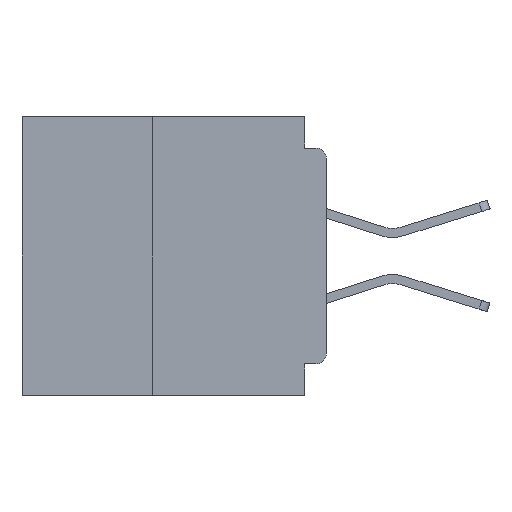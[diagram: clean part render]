
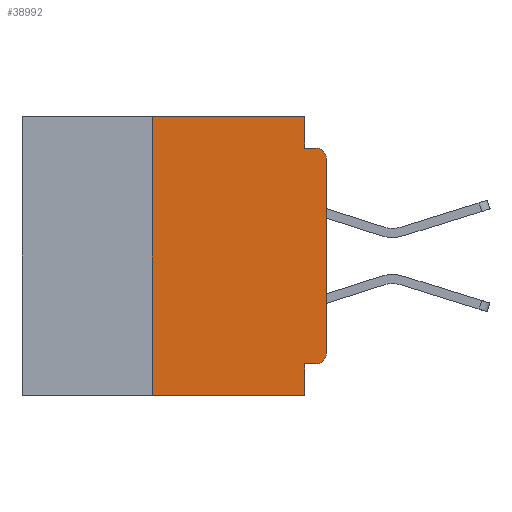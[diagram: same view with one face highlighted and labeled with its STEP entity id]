
A CAD part, left-side view. The second image highlights one B-rep face of the part: STEP entity #38992.
In plain terms, the highlighted planar face has unit normal (-1, 0, 0).
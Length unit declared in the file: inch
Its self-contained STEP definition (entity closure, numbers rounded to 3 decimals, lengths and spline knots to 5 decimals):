
#141 = CARTESIAN_POINT ( 'NONE',  ( 0., 0., -0.06 ) ) ;
#2053 = EDGE_CURVE ( 'NONE', #21252, #15218, #48424, .T. ) ;
#2383 = ORIENTED_EDGE ( 'NONE', *, *, #46104, .F. ) ;
#2386 = VERTEX_POINT ( 'NONE', #37650 ) ;
#2969 = DIRECTION ( 'NONE',  ( 0., 0., -1. ) ) ;
#3203 = AXIS2_PLACEMENT_3D ( 'NONE', #31301, #7996, #35089 ) ;
#5048 = VECTOR ( 'NONE', #17751, 39.37008 ) ;
#5997 = EDGE_CURVE ( 'NONE', #2386, #42788, #24803, .T. ) ;
#6348 = EDGE_CURVE ( 'NONE', #21252, #23633, #40868, .T. ) ;
#6538 = VECTOR ( 'NONE', #2969, 39.37008 ) ;
#7996 = DIRECTION ( 'NONE',  ( -1., 0., 0. ) ) ;
#8627 = CARTESIAN_POINT ( 'NONE',  ( 0., 0.031, -0.4 ) ) ;
#9634 = VERTEX_POINT ( 'NONE', #15767 ) ;
#10003 = CARTESIAN_POINT ( 'NONE',  ( 0., 0., 0. ) ) ;
#10216 = ORIENTED_EDGE ( 'NONE', *, *, #6348, .F. ) ;
#11369 = CARTESIAN_POINT ( 'NONE',  ( 0., 0.25, -0.4 ) ) ;
#11810 = PLANE ( 'NONE',  #15369 ) ;
#14421 = VECTOR ( 'NONE', #28930, 39.37008 ) ;
#14521 = ORIENTED_EDGE ( 'NONE', *, *, #5997, .F. ) ;
#14893 = CARTESIAN_POINT ( 'NONE',  ( 0., 0.25, 0. ) ) ;
#15218 = VERTEX_POINT ( 'NONE', #8627 ) ;
#15369 = AXIS2_PLACEMENT_3D ( 'NONE', #31027, #38784, #15764 ) ;
#15726 = LINE ( 'NONE', #18383, #6538 ) ;
#15750 = VERTEX_POINT ( 'NONE', #27182 ) ;
#15764 = DIRECTION ( 'NONE',  ( 0., 0., -1. ) ) ;
#15767 = CARTESIAN_POINT ( 'NONE',  ( 0., 0., -0.34 ) ) ;
#17426 = LINE ( 'NONE', #30052, #26524 ) ;
#17730 = ORIENTED_EDGE ( 'NONE', *, *, #43444, .T. ) ;
#17751 = DIRECTION ( 'NONE',  ( 0., 0., 1. ) ) ;
#18383 = CARTESIAN_POINT ( 'NONE',  ( 0., 0.031, -0.4 ) ) ;
#18812 = EDGE_CURVE ( 'NONE', #29042, #29140, #17426, .T. ) ;
#18917 = VECTOR ( 'NONE', #31744, 39.37008 ) ;
#19484 = EDGE_CURVE ( 'NONE', #15750, #29042, #28282, .T. ) ;
#21252 = VERTEX_POINT ( 'NONE', #33305 ) ;
#22038 = CARTESIAN_POINT ( 'NONE',  ( 0., 0.015, -0.06 ) ) ;
#23633 = VERTEX_POINT ( 'NONE', #14893 ) ;
#24329 = CARTESIAN_POINT ( 'NONE',  ( 0., 0.437, -0.4 ) ) ;
#24803 = LINE ( 'NONE', #25080, #14421 ) ;
#25080 = CARTESIAN_POINT ( 'NONE',  ( 0., 0., -0.355 ) ) ;
#25946 = DIRECTION ( 'NONE',  ( 0., 0., -1. ) ) ;
#26339 = ORIENTED_EDGE ( 'NONE', *, *, #38634, .T. ) ;
#26524 = VECTOR ( 'NONE', #45489, 39.37008 ) ;
#26985 = EDGE_CURVE ( 'NONE', #9634, #28193, #35965, .T. ) ;
#27071 = DIRECTION ( 'NONE',  ( 0., 0., 1. ) ) ;
#27182 = CARTESIAN_POINT ( 'NONE',  ( 0., 0.031, 0. ) ) ;
#27909 = CARTESIAN_POINT ( 'NONE',  ( 0., 0.437, 0. ) ) ;
#28193 = VERTEX_POINT ( 'NONE', #141 ) ;
#28212 = DIRECTION ( 'NONE',  ( 0., -1., 0. ) ) ;
#28242 = VECTOR ( 'NONE', #28212, 39.37008 ) ;
#28282 = LINE ( 'NONE', #49255, #37181 ) ;
#28299 = AXIS2_PLACEMENT_3D ( 'NONE', #22038, #48709, #25946 ) ;
#28930 = DIRECTION ( 'NONE',  ( 0., 1., 0. ) ) ;
#29042 = VERTEX_POINT ( 'NONE', #48665 ) ;
#29140 = VERTEX_POINT ( 'NONE', #37718 ) ;
#30052 = CARTESIAN_POINT ( 'NONE',  ( 0., 0., -0.045 ) ) ;
#31027 = CARTESIAN_POINT ( 'NONE',  ( 0., 0.437, 0. ) ) ;
#31301 = CARTESIAN_POINT ( 'NONE',  ( 0., 0.015, -0.34 ) ) ;
#31744 = DIRECTION ( 'NONE',  ( 0., -1., 0. ) ) ;
#33014 = CARTESIAN_POINT ( 'NONE',  ( 0., 0.031, -0.355 ) ) ;
#33305 = CARTESIAN_POINT ( 'NONE',  ( 0., 0.25, -0.4 ) ) ;
#33657 = FACE_OUTER_BOUND ( 'NONE', #40827, .T. ) ;
#34039 = ORIENTED_EDGE ( 'NONE', *, *, #47928, .F. ) ;
#35089 = DIRECTION ( 'NONE',  ( 0., 0., -1. ) ) ;
#35480 = ORIENTED_EDGE ( 'NONE', *, *, #18812, .F. ) ;
#35965 = LINE ( 'NONE', #10003, #5048 ) ;
#36112 = VECTOR ( 'NONE', #27071, 39.37008 ) ;
#36739 = ORIENTED_EDGE ( 'NONE', *, *, #2053, .T. ) ;
#37181 = VECTOR ( 'NONE', #37801, 39.37008 ) ;
#37650 = CARTESIAN_POINT ( 'NONE',  ( 0., 0.015, -0.355 ) ) ;
#37718 = CARTESIAN_POINT ( 'NONE',  ( 0., 0.015, -0.045 ) ) ;
#37801 = DIRECTION ( 'NONE',  ( 0., 0., -1. ) ) ;
#38634 = EDGE_CURVE ( 'NONE', #2386, #9634, #40239, .T. ) ;
#38784 = DIRECTION ( 'NONE',  ( 1., 0., 0. ) ) ;
#38992 = ADVANCED_FACE ( 'NONE', ( #33657 ), #11810, .F. ) ;
#39213 = CIRCLE ( 'NONE', #28299, 0.015 ) ;
#40239 = CIRCLE ( 'NONE', #3203, 0.015 ) ;
#40827 = EDGE_LOOP ( 'NONE', ( #48139, #17730, #35480, #49171, #2383, #10216, #36739, #34039, #14521, #26339 ) ) ;
#40868 = LINE ( 'NONE', #11369, #36112 ) ;
#42788 = VERTEX_POINT ( 'NONE', #33014 ) ;
#43444 = EDGE_CURVE ( 'NONE', #28193, #29140, #39213, .T. ) ;
#45489 = DIRECTION ( 'NONE',  ( 0., -1., 0. ) ) ;
#46104 = EDGE_CURVE ( 'NONE', #23633, #15750, #49396, .T. ) ;
#47928 = EDGE_CURVE ( 'NONE', #42788, #15218, #15726, .T. ) ;
#48139 = ORIENTED_EDGE ( 'NONE', *, *, #26985, .T. ) ;
#48424 = LINE ( 'NONE', #24329, #28242 ) ;
#48665 = CARTESIAN_POINT ( 'NONE',  ( 0., 0.031, -0.045 ) ) ;
#48709 = DIRECTION ( 'NONE',  ( -1., 0., 0. ) ) ;
#49171 = ORIENTED_EDGE ( 'NONE', *, *, #19484, .F. ) ;
#49255 = CARTESIAN_POINT ( 'NONE',  ( 0., 0.031, 0. ) ) ;
#49396 = LINE ( 'NONE', #27909, #18917 ) ;
